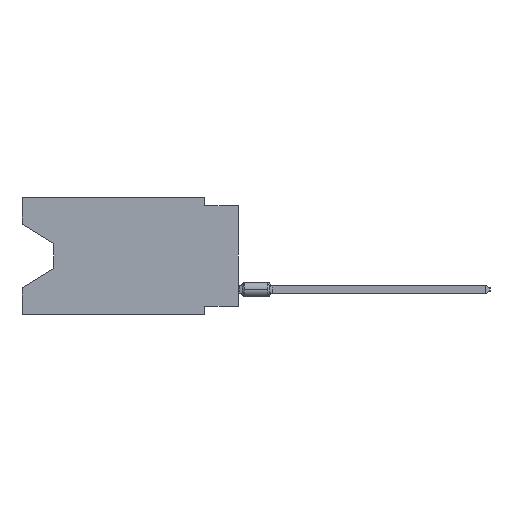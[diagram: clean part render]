
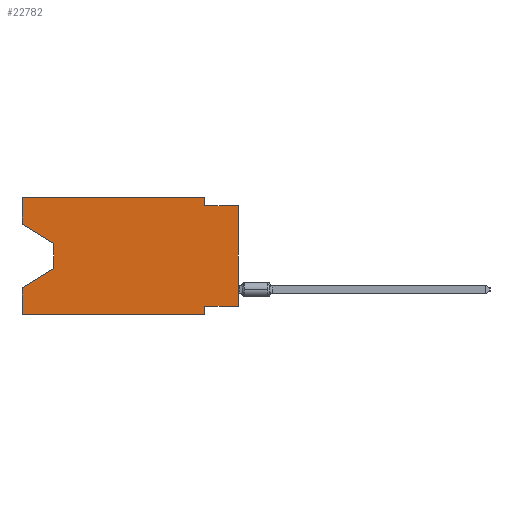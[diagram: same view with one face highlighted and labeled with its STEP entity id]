
A CAD part, left-side view. The second image highlights one B-rep face of the part: STEP entity #22782.
In plain terms, the highlighted planar face has unit normal (-1, 0, 0).
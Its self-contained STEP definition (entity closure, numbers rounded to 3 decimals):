
#1518 = EDGE_LOOP ( 'NONE', ( #41491, #42278, #43601, #34673, #40345, #40031, #38308, #13424, #32589, #32200, #40709, #16376 ) ) ;
#2983 = CARTESIAN_POINT ( 'NONE',  ( 0., 0., -0.635 ) ) ;
#3505 = CARTESIAN_POINT ( 'NONE',  ( 0., 2.54, -8.89 ) ) ;
#5170 = EDGE_CURVE ( 'NONE', #24766, #44150, #41287, .T. ) ;
#5500 = CARTESIAN_POINT ( 'NONE',  ( 0., 13.97, -5.385 ) ) ;
#6701 = DIRECTION ( 'NONE',  ( 0., 0., 1. ) ) ;
#6986 = DIRECTION ( 'NONE',  ( 0., 0., -1. ) ) ;
#7323 = EDGE_CURVE ( 'NONE', #41757, #44150, #51186, .T. ) ;
#8186 = LINE ( 'NONE', #48514, #9336 ) ;
#8260 = CARTESIAN_POINT ( 'NONE',  ( 0., 0., -8.255 ) ) ;
#8396 = VECTOR ( 'NONE', #27440, 1000. ) ;
#8856 = VECTOR ( 'NONE', #10998, 1000. ) ;
#9003 = CARTESIAN_POINT ( 'NONE',  ( 0., 16.383, -8.89 ) ) ;
#9291 = VECTOR ( 'NONE', #21115, 1000. ) ;
#9336 = VECTOR ( 'NONE', #41112, 1000. ) ;
#9583 = EDGE_CURVE ( 'NONE', #24686, #20288, #14604, .T. ) ;
#10050 = VERTEX_POINT ( 'NONE', #31631 ) ;
#10998 = DIRECTION ( 'NONE',  ( 0., -1., 0. ) ) ;
#12206 = LINE ( 'NONE', #8260, #36999 ) ;
#12336 = EDGE_CURVE ( 'NONE', #10050, #44174, #35070, .T. ) ;
#13424 = ORIENTED_EDGE ( 'NONE', *, *, #7323, .T. ) ;
#14604 = LINE ( 'NONE', #47546, #22452 ) ;
#14686 = CARTESIAN_POINT ( 'NONE',  ( 0., 16.383, 0. ) ) ;
#14946 = LINE ( 'NONE', #14686, #8856 ) ;
#15053 = DIRECTION ( 'NONE',  ( 0., 0., -1. ) ) ;
#16376 = ORIENTED_EDGE ( 'NONE', *, *, #20014, .F. ) ;
#16508 = CARTESIAN_POINT ( 'NONE',  ( 0., 0., -0.635 ) ) ;
#17160 = CARTESIAN_POINT ( 'NONE',  ( 0., 16.383, -2.038 ) ) ;
#17638 = EDGE_CURVE ( 'NONE', #24686, #44174, #20078, .T. ) ;
#17678 = VERTEX_POINT ( 'NONE', #17160 ) ;
#18315 = DIRECTION ( 'NONE',  ( 0., 0., -1. ) ) ;
#18942 = VECTOR ( 'NONE', #18315, 1000. ) ;
#20014 = EDGE_CURVE ( 'NONE', #17678, #29515, #33592, .T. ) ;
#20078 = LINE ( 'NONE', #9003, #9291 ) ;
#20288 = VERTEX_POINT ( 'NONE', #31713 ) ;
#21115 = DIRECTION ( 'NONE',  ( 0., -1., 0. ) ) ;
#21761 = VERTEX_POINT ( 'NONE', #5500 ) ;
#22021 = LINE ( 'NONE', #41799, #18942 ) ;
#22366 = VERTEX_POINT ( 'NONE', #26487 ) ;
#22452 = VECTOR ( 'NONE', #6701, 1000. ) ;
#22782 = ADVANCED_FACE ( 'NONE', ( #32396 ), #48504, .F. ) ;
#24686 = VERTEX_POINT ( 'NONE', #27825 ) ;
#24766 = VERTEX_POINT ( 'NONE', #24904 ) ;
#24904 = CARTESIAN_POINT ( 'NONE',  ( 0., 2.54, -0.635 ) ) ;
#26487 = CARTESIAN_POINT ( 'NONE',  ( 0., 13.97, -3.505 ) ) ;
#27435 = DIRECTION ( 'NONE',  ( 0., 0., 1. ) ) ;
#27440 = DIRECTION ( 'NONE',  ( 0., -0.855, -0.519 ) ) ;
#27825 = CARTESIAN_POINT ( 'NONE',  ( 0., 16.383, -8.89 ) ) ;
#28453 = DIRECTION ( 'NONE',  ( 1., 0., 0. ) ) ;
#29273 = VECTOR ( 'NONE', #15053, 1000. ) ;
#29515 = VERTEX_POINT ( 'NONE', #31515 ) ;
#29647 = CARTESIAN_POINT ( 'NONE',  ( 0., 16.383, 0. ) ) ;
#29898 = DIRECTION ( 'NONE',  ( 0., 0., 1. ) ) ;
#31009 = AXIS2_PLACEMENT_3D ( 'NONE', #33170, #28453, #32920 ) ;
#31515 = CARTESIAN_POINT ( 'NONE',  ( 0., 16.383, 0. ) ) ;
#31631 = CARTESIAN_POINT ( 'NONE',  ( 0., 2.54, -8.255 ) ) ;
#31713 = CARTESIAN_POINT ( 'NONE',  ( 0., 16.383, -6.852 ) ) ;
#32200 = ORIENTED_EDGE ( 'NONE', *, *, #49022, .F. ) ;
#32396 = FACE_OUTER_BOUND ( 'NONE', #1518, .T. ) ;
#32576 = DIRECTION ( 'NONE',  ( 0., -1., 0. ) ) ;
#32589 = ORIENTED_EDGE ( 'NONE', *, *, #5170, .F. ) ;
#32920 = DIRECTION ( 'NONE',  ( 0., 0., -1. ) ) ;
#33170 = CARTESIAN_POINT ( 'NONE',  ( 0., 16.383, 0. ) ) ;
#33592 = LINE ( 'NONE', #29647, #49192 ) ;
#34673 = ORIENTED_EDGE ( 'NONE', *, *, #9583, .F. ) ;
#35070 = LINE ( 'NONE', #51184, #29273 ) ;
#35345 = LINE ( 'NONE', #51455, #8396 ) ;
#36475 = EDGE_CURVE ( 'NONE', #22366, #21761, #43094, .T. ) ;
#36999 = VECTOR ( 'NONE', #51503, 1000. ) ;
#38308 = ORIENTED_EDGE ( 'NONE', *, *, #38799, .F. ) ;
#38799 = EDGE_CURVE ( 'NONE', #41757, #10050, #12206, .T. ) ;
#39037 = CARTESIAN_POINT ( 'NONE',  ( 0., 0., 0. ) ) ;
#39487 = VECTOR ( 'NONE', #6986, 1000. ) ;
#40031 = ORIENTED_EDGE ( 'NONE', *, *, #12336, .F. ) ;
#40345 = ORIENTED_EDGE ( 'NONE', *, *, #17638, .T. ) ;
#40709 = ORIENTED_EDGE ( 'NONE', *, *, #48819, .F. ) ;
#40711 = VECTOR ( 'NONE', #27435, 1000. ) ;
#41112 = DIRECTION ( 'NONE',  ( 0., 0.855, -0.519 ) ) ;
#41287 = LINE ( 'NONE', #16508, #44641 ) ;
#41491 = ORIENTED_EDGE ( 'NONE', *, *, #46840, .T. ) ;
#41757 = VERTEX_POINT ( 'NONE', #43807 ) ;
#41799 = CARTESIAN_POINT ( 'NONE',  ( 0., 2.54, 0. ) ) ;
#42278 = ORIENTED_EDGE ( 'NONE', *, *, #36475, .T. ) ;
#43079 = EDGE_CURVE ( 'NONE', #21761, #20288, #8186, .T. ) ;
#43094 = LINE ( 'NONE', #43621, #39487 ) ;
#43601 = ORIENTED_EDGE ( 'NONE', *, *, #43079, .T. ) ;
#43621 = CARTESIAN_POINT ( 'NONE',  ( 0., 13.97, -3.505 ) ) ;
#43807 = CARTESIAN_POINT ( 'NONE',  ( 0., 0., -8.255 ) ) ;
#44150 = VERTEX_POINT ( 'NONE', #2983 ) ;
#44174 = VERTEX_POINT ( 'NONE', #3505 ) ;
#44641 = VECTOR ( 'NONE', #32576, 1000. ) ;
#46840 = EDGE_CURVE ( 'NONE', #17678, #22366, #35345, .T. ) ;
#47546 = CARTESIAN_POINT ( 'NONE',  ( 0., 16.383, 0. ) ) ;
#48504 = PLANE ( 'NONE',  #31009 ) ;
#48514 = CARTESIAN_POINT ( 'NONE',  ( 0., 13.97, -5.385 ) ) ;
#48819 = EDGE_CURVE ( 'NONE', #29515, #51731, #14946, .T. ) ;
#49022 = EDGE_CURVE ( 'NONE', #51731, #24766, #22021, .T. ) ;
#49192 = VECTOR ( 'NONE', #29898, 1000. ) ;
#49874 = CARTESIAN_POINT ( 'NONE',  ( 0., 2.54, 0. ) ) ;
#51184 = CARTESIAN_POINT ( 'NONE',  ( 0., 2.54, -8.89 ) ) ;
#51186 = LINE ( 'NONE', #39037, #40711 ) ;
#51455 = CARTESIAN_POINT ( 'NONE',  ( 0., 16.383, -2.038 ) ) ;
#51503 = DIRECTION ( 'NONE',  ( 0., 1., 0. ) ) ;
#51731 = VERTEX_POINT ( 'NONE', #49874 ) ;
